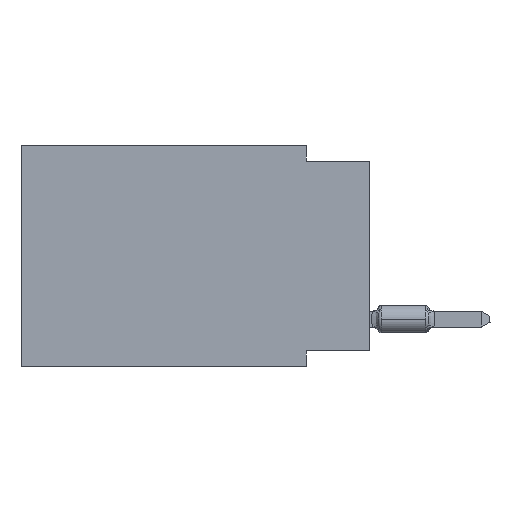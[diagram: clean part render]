
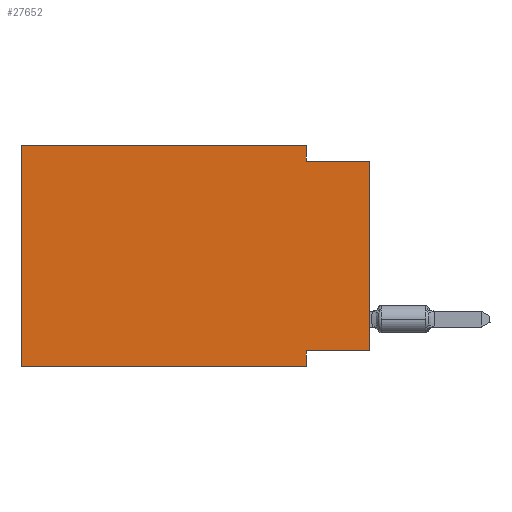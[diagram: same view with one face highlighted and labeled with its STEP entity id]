
A CAD part, left-side view. The second image highlights one B-rep face of the part: STEP entity #27652.
In plain terms, the highlighted planar face has unit normal (-1, 0, 0).
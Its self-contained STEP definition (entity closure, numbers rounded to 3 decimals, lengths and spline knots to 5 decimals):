
#1259 = CARTESIAN_POINT ( 'NONE',  ( 0., 0.1, -0.025 ) ) ;
#1679 = CARTESIAN_POINT ( 'NONE',  ( 0., 0.55, 0. ) ) ;
#3111 = ORIENTED_EDGE ( 'NONE', *, *, #87144, .F. ) ;
#3379 = DIRECTION ( 'NONE',  ( 0., 1., 0. ) ) ;
#4062 = LINE ( 'NONE', #1679, #81149 ) ;
#7863 = ORIENTED_EDGE ( 'NONE', *, *, #14278, .F. ) ;
#12207 = DIRECTION ( 'NONE',  ( 0., -1., 0. ) ) ;
#12930 = VERTEX_POINT ( 'NONE', #15902 ) ;
#13118 = VERTEX_POINT ( 'NONE', #13374 ) ;
#13374 = CARTESIAN_POINT ( 'NONE',  ( 0., 0., -0.025 ) ) ;
#13688 = CARTESIAN_POINT ( 'NONE',  ( 0., 0.1, 0. ) ) ;
#14278 = EDGE_CURVE ( 'NONE', #74881, #114909, #58082, .T. ) ;
#15902 = CARTESIAN_POINT ( 'NONE',  ( 0., 0., -0.325 ) ) ;
#16557 = VECTOR ( 'NONE', #76904, 39.37008 ) ;
#18643 = LINE ( 'NONE', #55441, #43402 ) ;
#18994 = CARTESIAN_POINT ( 'NONE',  ( 0., 0.1, -0.35 ) ) ;
#19772 = LINE ( 'NONE', #65048, #79956 ) ;
#19847 = CARTESIAN_POINT ( 'NONE',  ( 0., 0.55, 0. ) ) ;
#20446 = DIRECTION ( 'NONE',  ( 1., 0., 0. ) ) ;
#20900 = LINE ( 'NONE', #57698, #65720 ) ;
#21023 = VERTEX_POINT ( 'NONE', #29249 ) ;
#21056 = DIRECTION ( 'NONE',  ( 0., 0., -1. ) ) ;
#22035 = CARTESIAN_POINT ( 'NONE',  ( 0., 0.1, 0. ) ) ;
#25471 = LINE ( 'NONE', #22035, #16557 ) ;
#25689 = ORIENTED_EDGE ( 'NONE', *, *, #65861, .F. ) ;
#26134 = ORIENTED_EDGE ( 'NONE', *, *, #114786, .T. ) ;
#27005 = ORIENTED_EDGE ( 'NONE', *, *, #61054, .F. ) ;
#27448 = EDGE_CURVE ( 'NONE', #12930, #13118, #110940, .T. ) ;
#27652 = ADVANCED_FACE ( 'NONE', ( #94643 ), #56650, .F. ) ;
#29249 = CARTESIAN_POINT ( 'NONE',  ( 0., 0.1, -0.325 ) ) ;
#35588 = CARTESIAN_POINT ( 'NONE',  ( 0., 0., 0. ) ) ;
#36034 = AXIS2_PLACEMENT_3D ( 'NONE', #19847, #20446, #21056 ) ;
#37945 = DIRECTION ( 'NONE',  ( 0., -1., 0. ) ) ;
#43402 = VECTOR ( 'NONE', #37945, 39.37008 ) ;
#53351 = VECTOR ( 'NONE', #81992, 39.37008 ) ;
#53614 = VECTOR ( 'NONE', #75062, 39.37008 ) ;
#55187 = ORIENTED_EDGE ( 'NONE', *, *, #95265, .F. ) ;
#55441 = CARTESIAN_POINT ( 'NONE',  ( 0., 0., -0.025 ) ) ;
#56650 = PLANE ( 'NONE',  #36034 ) ;
#57698 = CARTESIAN_POINT ( 'NONE',  ( 0., 0., -0.325 ) ) ;
#57940 = EDGE_LOOP ( 'NONE', ( #79916, #3111, #64913, #7863, #55187, #26134, #27005, #25689 ) ) ;
#58082 = LINE ( 'NONE', #94873, #84104 ) ;
#61054 = EDGE_CURVE ( 'NONE', #21023, #74834, #76252, .T. ) ;
#64913 = ORIENTED_EDGE ( 'NONE', *, *, #102206, .F. ) ;
#65048 = CARTESIAN_POINT ( 'NONE',  ( 0., 0.55, -0.35 ) ) ;
#65720 = VECTOR ( 'NONE', #3379, 39.37008 ) ;
#65861 = EDGE_CURVE ( 'NONE', #12930, #21023, #20900, .T. ) ;
#74417 = CARTESIAN_POINT ( 'NONE',  ( 0., 0.55, 0. ) ) ;
#74834 = VERTEX_POINT ( 'NONE', #112381 ) ;
#74881 = VERTEX_POINT ( 'NONE', #74417 ) ;
#75062 = DIRECTION ( 'NONE',  ( 0., 0., -1. ) ) ;
#75210 = VERTEX_POINT ( 'NONE', #1259 ) ;
#76252 = LINE ( 'NONE', #18994, #53614 ) ;
#76904 = DIRECTION ( 'NONE',  ( 0., 0., -1. ) ) ;
#79916 = ORIENTED_EDGE ( 'NONE', *, *, #27448, .T. ) ;
#79956 = VECTOR ( 'NONE', #101231, 39.37008 ) ;
#81149 = VECTOR ( 'NONE', #85514, 39.37008 ) ;
#81992 = DIRECTION ( 'NONE',  ( 0., 0., 1. ) ) ;
#84104 = VECTOR ( 'NONE', #12207, 39.37008 ) ;
#85514 = DIRECTION ( 'NONE',  ( 0., 0., 1. ) ) ;
#87144 = EDGE_CURVE ( 'NONE', #75210, #13118, #18643, .T. ) ;
#94643 = FACE_OUTER_BOUND ( 'NONE', #57940, .T. ) ;
#94873 = CARTESIAN_POINT ( 'NONE',  ( 0., 0.55, 0. ) ) ;
#95265 = EDGE_CURVE ( 'NONE', #106127, #74881, #4062, .T. ) ;
#101231 = DIRECTION ( 'NONE',  ( 0., -1., 0. ) ) ;
#102206 = EDGE_CURVE ( 'NONE', #114909, #75210, #25471, .T. ) ;
#106127 = VERTEX_POINT ( 'NONE', #115021 ) ;
#110940 = LINE ( 'NONE', #35588, #53351 ) ;
#112381 = CARTESIAN_POINT ( 'NONE',  ( 0., 0.1, -0.35 ) ) ;
#114786 = EDGE_CURVE ( 'NONE', #106127, #74834, #19772, .T. ) ;
#114909 = VERTEX_POINT ( 'NONE', #13688 ) ;
#115021 = CARTESIAN_POINT ( 'NONE',  ( 0., 0.55, -0.35 ) ) ;
